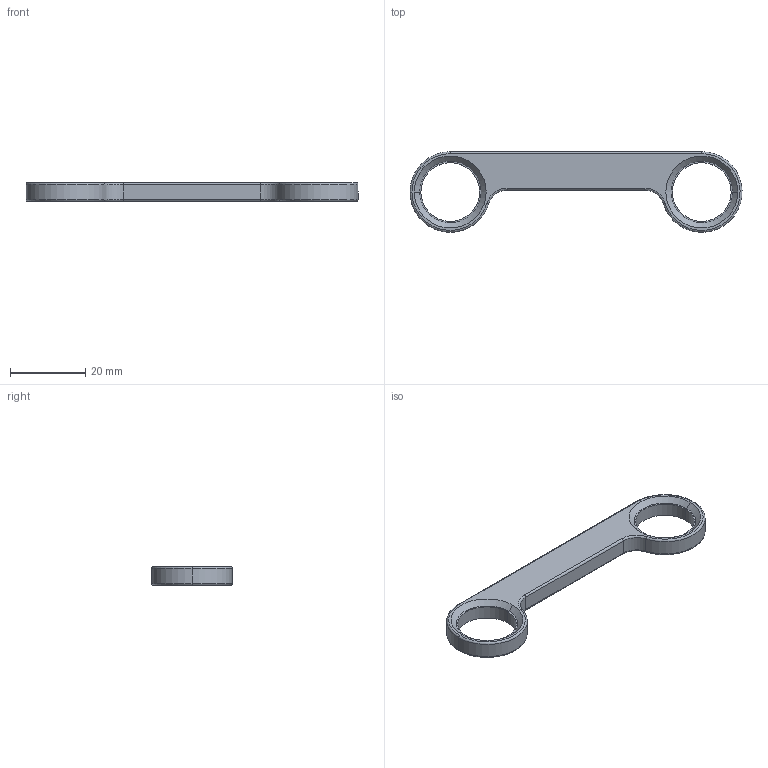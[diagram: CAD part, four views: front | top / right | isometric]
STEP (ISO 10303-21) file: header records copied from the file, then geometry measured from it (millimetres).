
FILE_DESCRIPTION (( 'STEP AP203' ), '1' );
FILE_NAME ('AF-WF-LR-PRT-007-STEP.STEP', '2020-07-22T09:32:32', ( '' ), ( '' ), 'SwSTEP 2.0', 'SolidWorks 2018', '' );
FILE_SCHEMA (( 'CONFIG_CONTROL_DESIGN' ));
Length unit declared in the file: inch
Products named in the file (1): AF-WF-LR-PRT-007-STEP
Bounding box: 88 x 21.31 x 4.95 mm (x, y, z)
Volume: 4041.4 mm3; surface area: 3068.1 mm2
Topology: 1 solids, 1 shells, 33 faces, 73 edges, 44 vertices
Faces by surface type: cylinder 13, torus 10, plane 6, cone 4
Entity records: 1012 total; most frequent: DIRECTION 191, CARTESIAN_POINT 151, ORIENTED_EDGE 146, AXIS2_PLACEMENT_3D 84, EDGE_CURVE 73, CIRCLE 50, VERTEX_POINT 44, EDGE_LOOP 39
